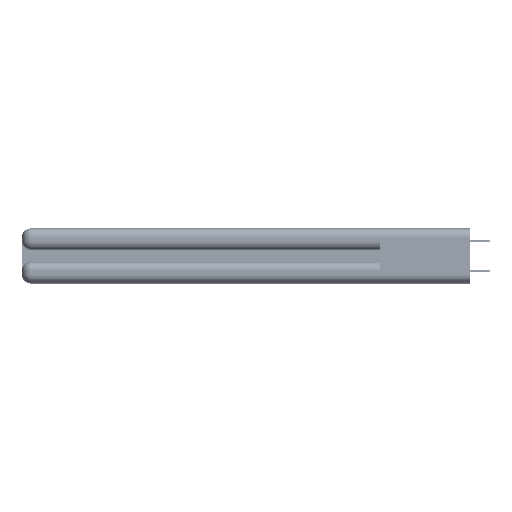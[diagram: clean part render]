
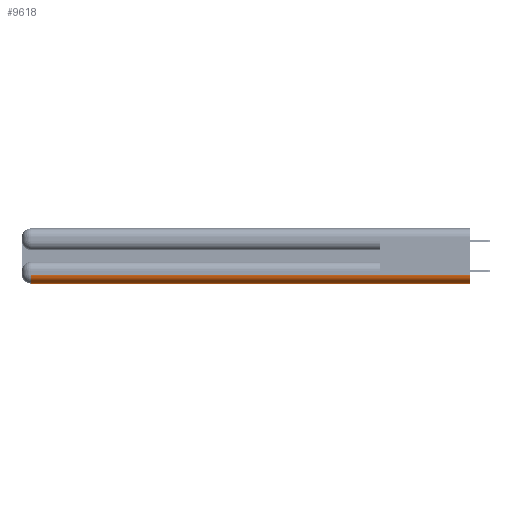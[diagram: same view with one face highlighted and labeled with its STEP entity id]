
A CAD part, left-side view. The second image highlights one B-rep face of the part: STEP entity #9618.
In plain terms, the highlighted cylindrical face has radius 1.524 mm (diameter 3.048 mm), a partial arc.
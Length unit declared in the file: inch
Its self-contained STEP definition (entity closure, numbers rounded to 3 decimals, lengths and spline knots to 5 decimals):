
#1488 = EDGE_CURVE ( 'NONE', #43431, #51145, #6581, .T. ) ;
#1980 = CARTESIAN_POINT ( 'NONE',  ( 0.06, 3., 0. ) ) ;
#3079 = ORIENTED_EDGE ( 'NONE', *, *, #17952, .F. ) ;
#3540 = ORIENTED_EDGE ( 'NONE', *, *, #41869, .F. ) ;
#4390 = CARTESIAN_POINT ( 'NONE',  ( 0.06, 0., 0.06 ) ) ;
#4831 = CARTESIAN_POINT ( 'NONE',  ( 0.06, 2.94, 0.06 ) ) ;
#5654 = VERTEX_POINT ( 'NONE', #25240 ) ;
#6423 = VECTOR ( 'NONE', #41521, 39.37008 ) ;
#6581 = CIRCLE ( 'NONE', #19218, 0.06 ) ;
#7298 = VECTOR ( 'NONE', #38366, 39.37008 ) ;
#9618 = ADVANCED_FACE ( 'NONE', ( #25889 ), #43107, .T. ) ;
#14709 = LINE ( 'NONE', #1980, #6423 ) ;
#17794 = CARTESIAN_POINT ( 'NONE',  ( 0.06, 0., 0.06 ) ) ;
#17952 = EDGE_CURVE ( 'NONE', #52758, #43431, #14709, .T. ) ;
#19218 = AXIS2_PLACEMENT_3D ( 'NONE', #4831, #39291, #40130 ) ;
#21140 = CARTESIAN_POINT ( 'NONE',  ( 0., 0., 0.06 ) ) ;
#21629 = DIRECTION ( 'NONE',  ( 0., 1., 0. ) ) ;
#21740 = DIRECTION ( 'NONE',  ( 0., 0., 1. ) ) ;
#25240 = CARTESIAN_POINT ( 'NONE',  ( 0., 0., 0.06 ) ) ;
#25889 = FACE_OUTER_BOUND ( 'NONE', #50823, .T. ) ;
#32104 = AXIS2_PLACEMENT_3D ( 'NONE', #17794, #34995, #21740 ) ;
#33822 = AXIS2_PLACEMENT_3D ( 'NONE', #4390, #21629, #49044 ) ;
#34144 = EDGE_CURVE ( 'NONE', #51145, #5654, #42596, .T. ) ;
#34502 = ORIENTED_EDGE ( 'NONE', *, *, #34144, .F. ) ;
#34995 = DIRECTION ( 'NONE',  ( 0., -1., 0. ) ) ;
#37997 = CARTESIAN_POINT ( 'NONE',  ( 0.06, 0., 0. ) ) ;
#38366 = DIRECTION ( 'NONE',  ( 0., -1., 0. ) ) ;
#39291 = DIRECTION ( 'NONE',  ( 0., 1., 0. ) ) ;
#40130 = DIRECTION ( 'NONE',  ( 0., 0., 1. ) ) ;
#40186 = CIRCLE ( 'NONE', #32104, 0.06 ) ;
#41521 = DIRECTION ( 'NONE',  ( 0., 1., 0. ) ) ;
#41869 = EDGE_CURVE ( 'NONE', #5654, #52758, #40186, .T. ) ;
#42596 = LINE ( 'NONE', #21140, #7298 ) ;
#43107 = CYLINDRICAL_SURFACE ( 'NONE', #33822, 0.06 ) ;
#43431 = VERTEX_POINT ( 'NONE', #54787 ) ;
#44368 = ORIENTED_EDGE ( 'NONE', *, *, #1488, .F. ) ;
#45302 = CARTESIAN_POINT ( 'NONE',  ( 0., 2.94, 0.06 ) ) ;
#49044 = DIRECTION ( 'NONE',  ( 0., 0., 1. ) ) ;
#50823 = EDGE_LOOP ( 'NONE', ( #3540, #34502, #44368, #3079 ) ) ;
#51145 = VERTEX_POINT ( 'NONE', #45302 ) ;
#52758 = VERTEX_POINT ( 'NONE', #37997 ) ;
#54787 = CARTESIAN_POINT ( 'NONE',  ( 0.06, 2.94, 0. ) ) ;
